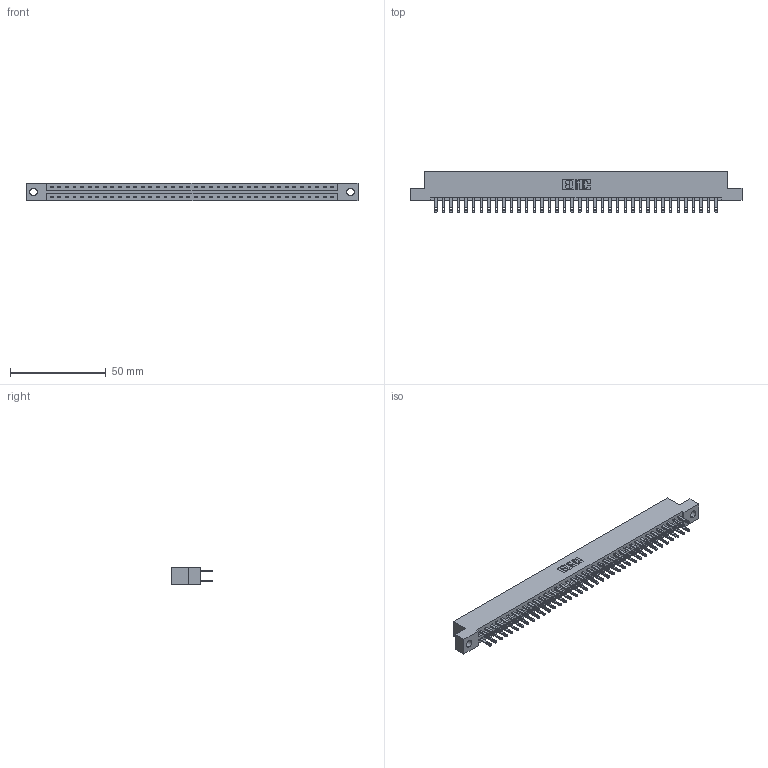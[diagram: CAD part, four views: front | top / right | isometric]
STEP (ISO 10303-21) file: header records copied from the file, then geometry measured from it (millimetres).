
FILE_DESCRIPTION (( 'STEP AP203' ), '1' );
FILE_NAME ('887-076-500-204.STEP', '2020-09-21T03:51:45', ( '' ), ( '' ), 'SwSTEP 2.0', 'SolidWorks 2020', '' );
FILE_SCHEMA (( 'CONFIG_CONTROL_DESIGN' ));
Length unit declared in the file: inch
Products named in the file (3): 887-076-500-204; 837 Part_Flush Mounting Lugs - 0.156 Dia-TH; 345-292-001_345-293-100
Assembly tree (77 placements, depth 2):
  887-076-500-204
    837 Part_Flush Mounting Lugs - 0.156 Dia-TH
    345-292-001_345-293-100  x76
Bounding box: 173.58 x 21.85 x 9.4 mm (x, y, z)
Volume: 18384.8 mm3; surface area: 21385.8 mm2
Topology: 77 solids, 77 shells, 3914 faces, 11939 edges, 7958 vertices
Faces by surface type: plane 2502, cylinder 1412
Entity records: 29913 total; most frequent: CARTESIAN_POINT 5042, ORIENTED_EDGE 4978, DIRECTION 4297, EDGE_CURVE 2489, LINE 2357, VECTOR 2357, VERTEX_POINT 1658, AXIS2_PLACEMENT_3D 970
